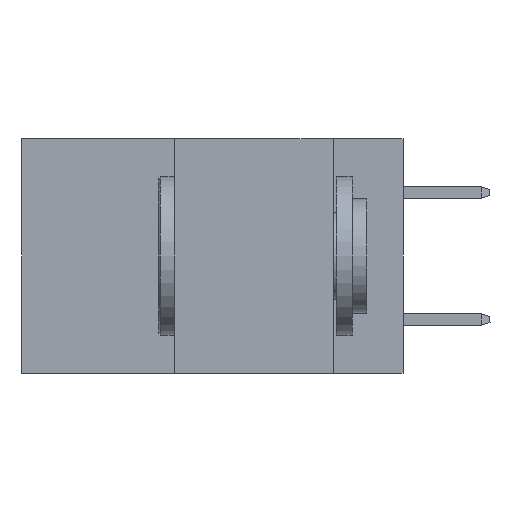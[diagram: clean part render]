
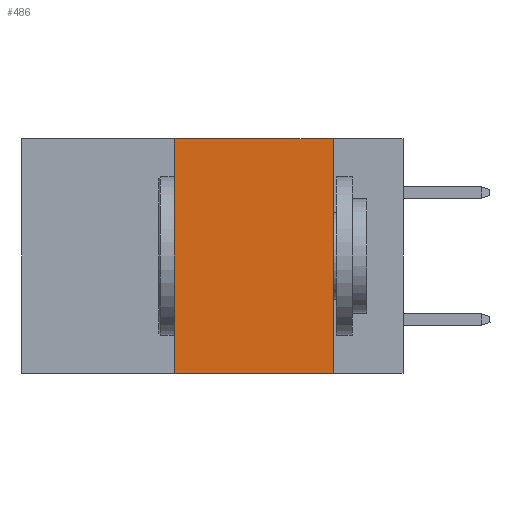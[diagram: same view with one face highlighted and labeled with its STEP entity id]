
A CAD part, left-side view. The second image highlights one B-rep face of the part: STEP entity #486.
In plain terms, the highlighted planar face has unit normal (-1, 0, 0).
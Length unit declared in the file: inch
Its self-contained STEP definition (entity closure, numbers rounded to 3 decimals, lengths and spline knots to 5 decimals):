
#30 = EDGE_CURVE ( 'NONE', #6990, #6620, #3738, .T. ) ;
#229 = CARTESIAN_POINT ( 'NONE',  ( 0., 0.6, -0.37 ) ) ;
#486 = ADVANCED_FACE ( 'NONE', ( #2439 ), #3660, .F. ) ;
#659 = VECTOR ( 'NONE', #7968, 39.37008 ) ;
#1909 = LINE ( 'NONE', #6816, #659 ) ;
#2439 = FACE_OUTER_BOUND ( 'NONE', #6519, .T. ) ;
#3278 = ORIENTED_EDGE ( 'NONE', *, *, #12497, .F. ) ;
#3660 = PLANE ( 'NONE',  #5255 ) ;
#3738 = LINE ( 'NONE', #7767, #11965 ) ;
#4369 = LINE ( 'NONE', #229, #12291 ) ;
#5255 = AXIS2_PLACEMENT_3D ( 'NONE', #10501, #9509, #11555 ) ;
#5586 = EDGE_CURVE ( 'NONE', #6386, #8719, #4369, .T. ) ;
#5759 = CARTESIAN_POINT ( 'NONE',  ( 0., 0.36, -0.37 ) ) ;
#5998 = ORIENTED_EDGE ( 'NONE', *, *, #11553, .F. ) ;
#6124 = DIRECTION ( 'NONE',  ( 0., -1., 0. ) ) ;
#6386 = VERTEX_POINT ( 'NONE', #5759 ) ;
#6519 = EDGE_LOOP ( 'NONE', ( #3278, #9928, #5998, #9503 ) ) ;
#6620 = VERTEX_POINT ( 'NONE', #6975 ) ;
#6816 = CARTESIAN_POINT ( 'NONE',  ( 0., 0.36, 0. ) ) ;
#6975 = CARTESIAN_POINT ( 'NONE',  ( 0., 0.11, 0. ) ) ;
#6990 = VERTEX_POINT ( 'NONE', #11019 ) ;
#7767 = CARTESIAN_POINT ( 'NONE',  ( 0., 0.6, 0. ) ) ;
#7968 = DIRECTION ( 'NONE',  ( 0., 0., 1. ) ) ;
#8333 = LINE ( 'NONE', #11367, #12925 ) ;
#8719 = VERTEX_POINT ( 'NONE', #10033 ) ;
#9503 = ORIENTED_EDGE ( 'NONE', *, *, #5586, .T. ) ;
#9509 = DIRECTION ( 'NONE',  ( 1., 0., 0. ) ) ;
#9573 = DIRECTION ( 'NONE',  ( 0., -1., 0. ) ) ;
#9928 = ORIENTED_EDGE ( 'NONE', *, *, #30, .F. ) ;
#10033 = CARTESIAN_POINT ( 'NONE',  ( 0., 0.11, -0.37 ) ) ;
#10312 = DIRECTION ( 'NONE',  ( 0., 0., -1. ) ) ;
#10501 = CARTESIAN_POINT ( 'NONE',  ( 0., 0.6, 0. ) ) ;
#11019 = CARTESIAN_POINT ( 'NONE',  ( 0., 0.36, 0. ) ) ;
#11367 = CARTESIAN_POINT ( 'NONE',  ( 0., 0.11, 0. ) ) ;
#11553 = EDGE_CURVE ( 'NONE', #6386, #6990, #1909, .T. ) ;
#11555 = DIRECTION ( 'NONE',  ( 0., 0., -1. ) ) ;
#11965 = VECTOR ( 'NONE', #9573, 39.37008 ) ;
#12291 = VECTOR ( 'NONE', #6124, 39.37008 ) ;
#12497 = EDGE_CURVE ( 'NONE', #6620, #8719, #8333, .T. ) ;
#12925 = VECTOR ( 'NONE', #10312, 39.37008 ) ;
